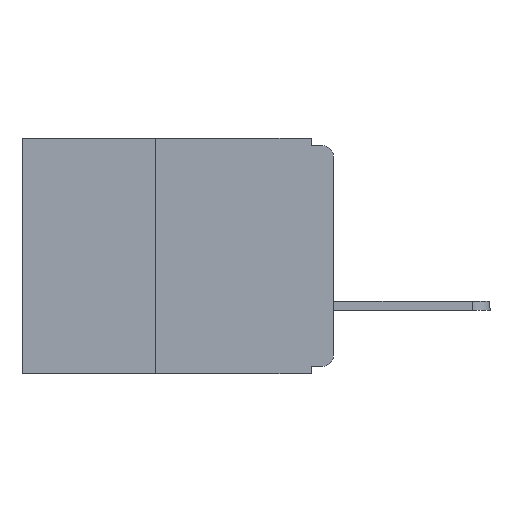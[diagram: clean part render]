
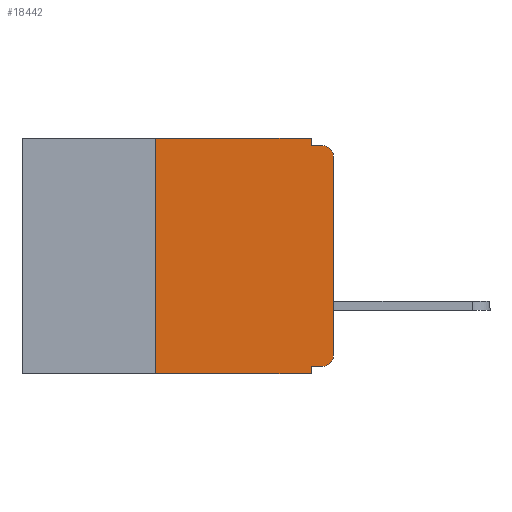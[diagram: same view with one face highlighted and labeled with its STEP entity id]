
A CAD part, left-side view. The second image highlights one B-rep face of the part: STEP entity #18442.
In plain terms, the highlighted planar face has unit normal (-1, 0, 0).
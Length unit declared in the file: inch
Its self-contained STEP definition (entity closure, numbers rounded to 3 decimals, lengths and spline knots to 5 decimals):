
#88 = DIRECTION ( 'NONE',  ( 0., 0., 1. ) ) ;
#711 = CARTESIAN_POINT ( 'NONE',  ( 0., 0.015, -0.305 ) ) ;
#1269 = AXIS2_PLACEMENT_3D ( 'NONE', #28344, #12240, #31061 ) ;
#2086 = DIRECTION ( 'NONE',  ( 0., 0., -1. ) ) ;
#3477 = DIRECTION ( 'NONE',  ( 0., 0., -1. ) ) ;
#4538 = ORIENTED_EDGE ( 'NONE', *, *, #28004, .T. ) ;
#5966 = EDGE_CURVE ( 'NONE', #24511, #29853, #26994, .T. ) ;
#6036 = LINE ( 'NONE', #26771, #13212 ) ;
#6422 = CARTESIAN_POINT ( 'NONE',  ( 0., 0.015, -0.01 ) ) ;
#6506 = CARTESIAN_POINT ( 'NONE',  ( 0., 0.015, -0.32 ) ) ;
#6595 = VECTOR ( 'NONE', #20710, 39.37008 ) ;
#6647 = LINE ( 'NONE', #11055, #20128 ) ;
#7307 = CARTESIAN_POINT ( 'NONE',  ( 0., 0., -0.025 ) ) ;
#9506 = AXIS2_PLACEMENT_3D ( 'NONE', #31758, #18286, #2086 ) ;
#10871 = ORIENTED_EDGE ( 'NONE', *, *, #11163, .T. ) ;
#11055 = CARTESIAN_POINT ( 'NONE',  ( 0., 0., -0.32 ) ) ;
#11163 = EDGE_CURVE ( 'NONE', #31740, #33939, #23456, .T. ) ;
#11314 = ORIENTED_EDGE ( 'NONE', *, *, #24167, .F. ) ;
#11551 = VECTOR ( 'NONE', #29573, 39.37008 ) ;
#12240 = DIRECTION ( 'NONE',  ( -1., 0., 0. ) ) ;
#12668 = VECTOR ( 'NONE', #16590, 39.37008 ) ;
#13212 = VECTOR ( 'NONE', #13336, 39.37008 ) ;
#13336 = DIRECTION ( 'NONE',  ( 0., -1., 0. ) ) ;
#13350 = CIRCLE ( 'NONE', #1269, 0.015 ) ;
#13854 = FACE_OUTER_BOUND ( 'NONE', #18290, .T. ) ;
#13881 = CARTESIAN_POINT ( 'NONE',  ( 0., 0.25, -0.33 ) ) ;
#14405 = VECTOR ( 'NONE', #22517, 39.37008 ) ;
#14507 = VERTEX_POINT ( 'NONE', #31543 ) ;
#14979 = ORIENTED_EDGE ( 'NONE', *, *, #34763, .F. ) ;
#15610 = PLANE ( 'NONE',  #9506 ) ;
#16590 = DIRECTION ( 'NONE',  ( 0., 0., 1. ) ) ;
#16736 = DIRECTION ( 'NONE',  ( 0., 0., -1. ) ) ;
#17017 = EDGE_CURVE ( 'NONE', #32687, #30661, #27868, .T. ) ;
#17336 = ORIENTED_EDGE ( 'NONE', *, *, #24119, .T. ) ;
#17556 = CIRCLE ( 'NONE', #27074, 0.015 ) ;
#18286 = DIRECTION ( 'NONE',  ( 1., 0., 0. ) ) ;
#18290 = EDGE_LOOP ( 'NONE', ( #10871, #28635, #22824, #23464, #31422, #33677, #17336, #11314, #14979, #4538 ) ) ;
#18442 = ADVANCED_FACE ( 'NONE', ( #13854 ), #15610, .F. ) ;
#19135 = DIRECTION ( 'NONE',  ( 0., 1., 0. ) ) ;
#19558 = EDGE_CURVE ( 'NONE', #33939, #30661, #13350, .T. ) ;
#19659 = DIRECTION ( 'NONE',  ( -1., 0., 0. ) ) ;
#20128 = VECTOR ( 'NONE', #19135, 39.37008 ) ;
#20710 = DIRECTION ( 'NONE',  ( 0., -1., 0. ) ) ;
#20828 = CARTESIAN_POINT ( 'NONE',  ( 0., 0.437, 0. ) ) ;
#20937 = LINE ( 'NONE', #20828, #6595 ) ;
#21219 = EDGE_CURVE ( 'NONE', #14507, #32687, #22943, .T. ) ;
#21600 = CARTESIAN_POINT ( 'NONE',  ( 0., 0.031, -0.33 ) ) ;
#21613 = VERTEX_POINT ( 'NONE', #31807 ) ;
#22517 = DIRECTION ( 'NONE',  ( 0., -1., 0. ) ) ;
#22624 = VECTOR ( 'NONE', #88, 39.37008 ) ;
#22824 = ORIENTED_EDGE ( 'NONE', *, *, #17017, .F. ) ;
#22942 = CARTESIAN_POINT ( 'NONE',  ( 0., 0.031, -0.01 ) ) ;
#22943 = LINE ( 'NONE', #24764, #29203 ) ;
#23456 = LINE ( 'NONE', #24463, #22624 ) ;
#23464 = ORIENTED_EDGE ( 'NONE', *, *, #21219, .F. ) ;
#24119 = EDGE_CURVE ( 'NONE', #24511, #26329, #6036, .T. ) ;
#24167 = EDGE_CURVE ( 'NONE', #21613, #26329, #33026, .T. ) ;
#24178 = CARTESIAN_POINT ( 'NONE',  ( 0., 0., -0.305 ) ) ;
#24463 = CARTESIAN_POINT ( 'NONE',  ( 0., 0., 0. ) ) ;
#24511 = VERTEX_POINT ( 'NONE', #25688 ) ;
#24764 = CARTESIAN_POINT ( 'NONE',  ( 0., 0.031, 0. ) ) ;
#25562 = CARTESIAN_POINT ( 'NONE',  ( 0., 0.031, -0.33 ) ) ;
#25688 = CARTESIAN_POINT ( 'NONE',  ( 0., 0.25, -0.33 ) ) ;
#26329 = VERTEX_POINT ( 'NONE', #25562 ) ;
#26771 = CARTESIAN_POINT ( 'NONE',  ( 0., 0.437, -0.33 ) ) ;
#26994 = LINE ( 'NONE', #13881, #12668 ) ;
#27074 = AXIS2_PLACEMENT_3D ( 'NONE', #711, #19659, #3477 ) ;
#27217 = CARTESIAN_POINT ( 'NONE',  ( 0., 0.25, 0. ) ) ;
#27774 = CARTESIAN_POINT ( 'NONE',  ( 0., 0., -0.01 ) ) ;
#27868 = LINE ( 'NONE', #27774, #14405 ) ;
#28004 = EDGE_CURVE ( 'NONE', #31342, #31740, #17556, .T. ) ;
#28300 = EDGE_CURVE ( 'NONE', #29853, #14507, #20937, .T. ) ;
#28344 = CARTESIAN_POINT ( 'NONE',  ( 0., 0.015, -0.025 ) ) ;
#28635 = ORIENTED_EDGE ( 'NONE', *, *, #19558, .T. ) ;
#29203 = VECTOR ( 'NONE', #16736, 39.37008 ) ;
#29573 = DIRECTION ( 'NONE',  ( 0., 0., -1. ) ) ;
#29853 = VERTEX_POINT ( 'NONE', #27217 ) ;
#30661 = VERTEX_POINT ( 'NONE', #6422 ) ;
#31061 = DIRECTION ( 'NONE',  ( 0., 0., -1. ) ) ;
#31342 = VERTEX_POINT ( 'NONE', #6506 ) ;
#31422 = ORIENTED_EDGE ( 'NONE', *, *, #28300, .F. ) ;
#31543 = CARTESIAN_POINT ( 'NONE',  ( 0., 0.031, 0. ) ) ;
#31740 = VERTEX_POINT ( 'NONE', #24178 ) ;
#31758 = CARTESIAN_POINT ( 'NONE',  ( 0., 0.437, 0. ) ) ;
#31807 = CARTESIAN_POINT ( 'NONE',  ( 0., 0.031, -0.32 ) ) ;
#32687 = VERTEX_POINT ( 'NONE', #22942 ) ;
#33026 = LINE ( 'NONE', #21600, #11551 ) ;
#33677 = ORIENTED_EDGE ( 'NONE', *, *, #5966, .F. ) ;
#33939 = VERTEX_POINT ( 'NONE', #7307 ) ;
#34763 = EDGE_CURVE ( 'NONE', #31342, #21613, #6647, .T. ) ;
